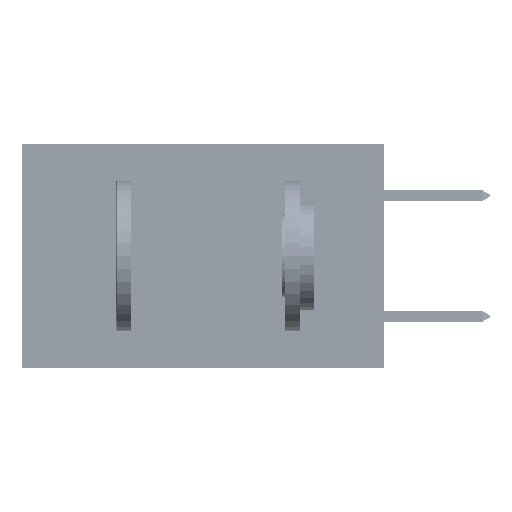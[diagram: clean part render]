
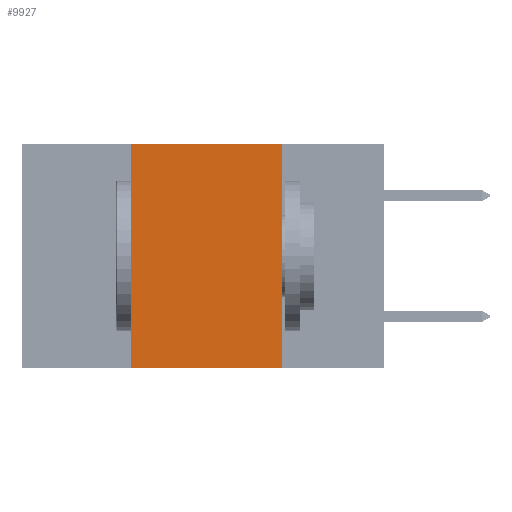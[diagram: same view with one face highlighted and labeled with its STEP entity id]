
A CAD part, left-side view. The second image highlights one B-rep face of the part: STEP entity #9927.
In plain terms, the highlighted planar face has unit normal (-1, 0, 0).
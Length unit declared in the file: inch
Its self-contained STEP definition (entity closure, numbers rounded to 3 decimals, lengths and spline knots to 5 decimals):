
#373 = CARTESIAN_POINT ( 'NONE',  ( 0., 0.17, 0. ) ) ;
#964 = CARTESIAN_POINT ( 'NONE',  ( 0., 0.6, 0. ) ) ;
#4031 = VERTEX_POINT ( 'NONE', #26549 ) ;
#4136 = EDGE_CURVE ( 'NONE', #4031, #33632, #46108, .T. ) ;
#8054 = DIRECTION ( 'NONE',  ( 1., 0., 0. ) ) ;
#9914 = EDGE_LOOP ( 'NONE', ( #16659, #36555, #32634, #29182 ) ) ;
#9927 = ADVANCED_FACE ( 'NONE', ( #42003 ), #39604, .F. ) ;
#10741 = DIRECTION ( 'NONE',  ( 0., 0., 1. ) ) ;
#11316 = EDGE_CURVE ( 'NONE', #4031, #44134, #25894, .T. ) ;
#12307 = VECTOR ( 'NONE', #21173, 39.37008 ) ;
#14829 = VECTOR ( 'NONE', #10741, 39.37008 ) ;
#15540 = CARTESIAN_POINT ( 'NONE',  ( 0., 0.42, 0. ) ) ;
#16200 = EDGE_CURVE ( 'NONE', #44134, #35483, #20276, .T. ) ;
#16659 = ORIENTED_EDGE ( 'NONE', *, *, #30276, .F. ) ;
#18429 = AXIS2_PLACEMENT_3D ( 'NONE', #32233, #8054, #19859 ) ;
#19124 = LINE ( 'NONE', #49352, #36944 ) ;
#19859 = DIRECTION ( 'NONE',  ( 0., 0., -1. ) ) ;
#20276 = LINE ( 'NONE', #964, #12307 ) ;
#21173 = DIRECTION ( 'NONE',  ( 0., -1., 0. ) ) ;
#25894 = LINE ( 'NONE', #34441, #14829 ) ;
#26549 = CARTESIAN_POINT ( 'NONE',  ( 0., 0.42, -0.37 ) ) ;
#27735 = DIRECTION ( 'NONE',  ( 0., -1., 0. ) ) ;
#29182 = ORIENTED_EDGE ( 'NONE', *, *, #4136, .T. ) ;
#30276 = EDGE_CURVE ( 'NONE', #35483, #33632, #19124, .T. ) ;
#30779 = VECTOR ( 'NONE', #27735, 39.37008 ) ;
#32233 = CARTESIAN_POINT ( 'NONE',  ( 0., 0.6, 0. ) ) ;
#32634 = ORIENTED_EDGE ( 'NONE', *, *, #11316, .F. ) ;
#33632 = VERTEX_POINT ( 'NONE', #38627 ) ;
#34441 = CARTESIAN_POINT ( 'NONE',  ( 0., 0.42, 0. ) ) ;
#35483 = VERTEX_POINT ( 'NONE', #373 ) ;
#36555 = ORIENTED_EDGE ( 'NONE', *, *, #16200, .F. ) ;
#36944 = VECTOR ( 'NONE', #45569, 39.37008 ) ;
#38627 = CARTESIAN_POINT ( 'NONE',  ( 0., 0.17, -0.37 ) ) ;
#39604 = PLANE ( 'NONE',  #18429 ) ;
#42003 = FACE_OUTER_BOUND ( 'NONE', #9914, .T. ) ;
#44134 = VERTEX_POINT ( 'NONE', #15540 ) ;
#45569 = DIRECTION ( 'NONE',  ( 0., 0., -1. ) ) ;
#46108 = LINE ( 'NONE', #46938, #30779 ) ;
#46938 = CARTESIAN_POINT ( 'NONE',  ( 0., 0.6, -0.37 ) ) ;
#49352 = CARTESIAN_POINT ( 'NONE',  ( 0., 0.17, 0. ) ) ;
